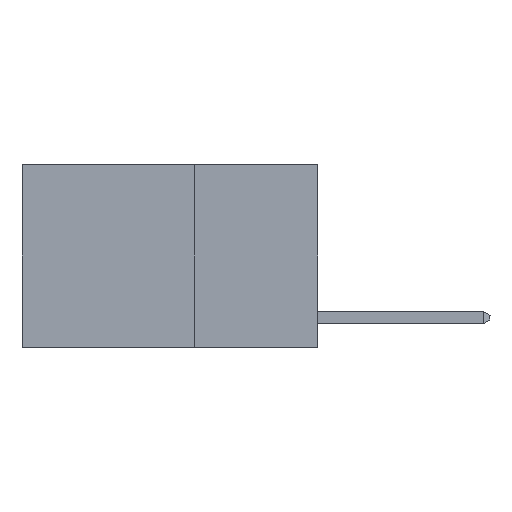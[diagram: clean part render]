
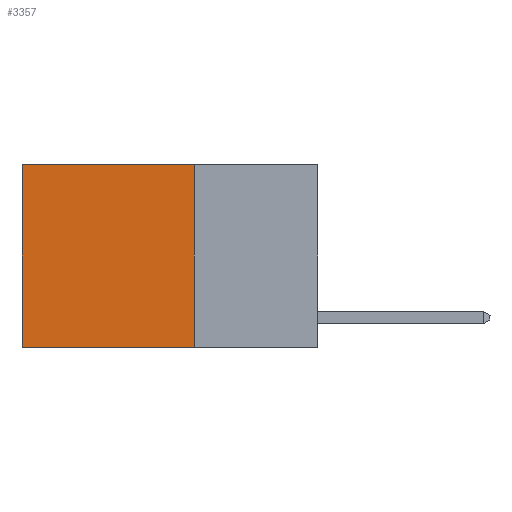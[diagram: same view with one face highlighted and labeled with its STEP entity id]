
A CAD part, left-side view. The second image highlights one B-rep face of the part: STEP entity #3357.
In plain terms, the highlighted planar face has unit normal (-1, 0, 0).
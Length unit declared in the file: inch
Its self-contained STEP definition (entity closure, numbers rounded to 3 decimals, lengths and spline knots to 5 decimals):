
#512 = LINE ( 'NONE', #2823, #6215 ) ;
#813 = PLANE ( 'NONE',  #3192 ) ;
#915 = CARTESIAN_POINT ( 'NONE',  ( 0.2625, 0.25, -0.37 ) ) ;
#1100 = VECTOR ( 'NONE', #4325, 39.37008 ) ;
#1299 = DIRECTION ( 'NONE',  ( 0., 1., 0. ) ) ;
#1502 = VERTEX_POINT ( 'NONE', #5405 ) ;
#1742 = DIRECTION ( 'NONE',  ( 0., 1., 0. ) ) ;
#1820 = EDGE_LOOP ( 'NONE', ( #4227, #3712, #6206, #2469 ) ) ;
#1927 = EDGE_CURVE ( 'NONE', #1502, #6936, #4467, .T. ) ;
#2324 = EDGE_CURVE ( 'NONE', #4648, #6936, #512, .T. ) ;
#2354 = DIRECTION ( 'NONE',  ( 1., 0., 0. ) ) ;
#2469 = ORIENTED_EDGE ( 'NONE', *, *, #6084, .T. ) ;
#2823 = CARTESIAN_POINT ( 'NONE',  ( 0.2625, 0.25, -0.37 ) ) ;
#3081 = DIRECTION ( 'NONE',  ( 0., 0., -1. ) ) ;
#3192 = AXIS2_PLACEMENT_3D ( 'NONE', #8723, #2354, #3081 ) ;
#3235 = CARTESIAN_POINT ( 'NONE',  ( 0.2625, 0.25, 0. ) ) ;
#3357 = ADVANCED_FACE ( 'NONE', ( #7872 ), #813, .F. ) ;
#3712 = ORIENTED_EDGE ( 'NONE', *, *, #2324, .F. ) ;
#4227 = ORIENTED_EDGE ( 'NONE', *, *, #1927, .T. ) ;
#4280 = CARTESIAN_POINT ( 'NONE',  ( 0.2625, 0.6, -0.37 ) ) ;
#4325 = DIRECTION ( 'NONE',  ( 0., 0., -1. ) ) ;
#4467 = LINE ( 'NONE', #8033, #1100 ) ;
#4648 = VERTEX_POINT ( 'NONE', #915 ) ;
#5405 = CARTESIAN_POINT ( 'NONE',  ( 0.2625, 0.6, 0. ) ) ;
#6032 = LINE ( 'NONE', #8213, #6042 ) ;
#6042 = VECTOR ( 'NONE', #1742, 39.37008 ) ;
#6084 = EDGE_CURVE ( 'NONE', #7585, #1502, #6032, .T. ) ;
#6206 = ORIENTED_EDGE ( 'NONE', *, *, #9152, .F. ) ;
#6215 = VECTOR ( 'NONE', #1299, 39.37008 ) ;
#6830 = DIRECTION ( 'NONE',  ( 0., 0., -1. ) ) ;
#6936 = VERTEX_POINT ( 'NONE', #4280 ) ;
#7046 = CARTESIAN_POINT ( 'NONE',  ( 0.2625, 0.25, 0. ) ) ;
#7585 = VERTEX_POINT ( 'NONE', #7046 ) ;
#7793 = VECTOR ( 'NONE', #6830, 39.37008 ) ;
#7872 = FACE_OUTER_BOUND ( 'NONE', #1820, .T. ) ;
#8033 = CARTESIAN_POINT ( 'NONE',  ( 0.2625, 0.6, 0. ) ) ;
#8075 = LINE ( 'NONE', #3235, #7793 ) ;
#8213 = CARTESIAN_POINT ( 'NONE',  ( 0.2625, 0.25, 0. ) ) ;
#8723 = CARTESIAN_POINT ( 'NONE',  ( 0.2625, 0.25, 0. ) ) ;
#9152 = EDGE_CURVE ( 'NONE', #7585, #4648, #8075, .T. ) ;
